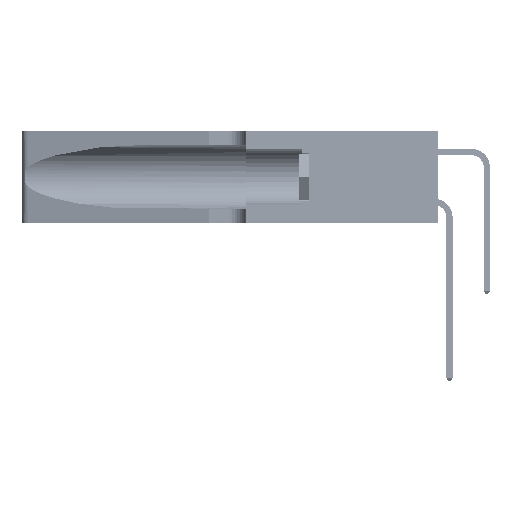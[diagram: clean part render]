
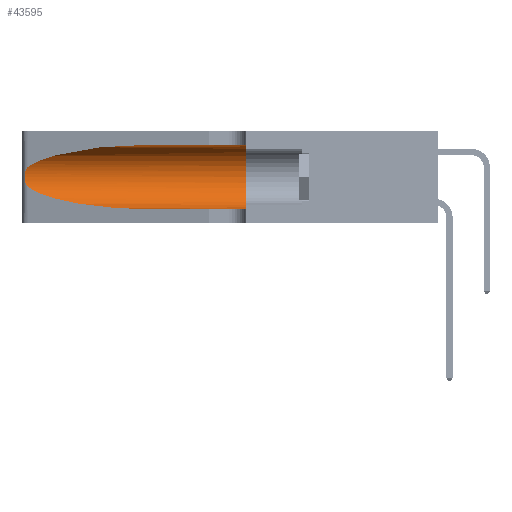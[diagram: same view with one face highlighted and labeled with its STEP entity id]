
A CAD part, left-side view. The second image highlights one B-rep face of the part: STEP entity #43595.
In plain terms, the highlighted cylindrical face has radius 3.308 mm (diameter 6.617 mm), a partial arc.
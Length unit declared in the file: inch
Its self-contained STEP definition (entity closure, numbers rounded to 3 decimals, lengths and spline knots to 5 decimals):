
#2756 = DIRECTION ( 'NONE',  ( 0., -1., 0. ) ) ;
#2828 = CARTESIAN_POINT ( 'NONE',  ( 0.26075, 1.23896, 0.19203 ) ) ;
#2876 = ORIENTED_EDGE ( 'NONE', *, *, #34880, .T. ) ;
#3377 = CARTESIAN_POINT ( 'NONE',  ( 0.2373, 1.15595, 0.28018 ) ) ;
#5323 = DIRECTION ( 'NONE',  ( 0., 1., 0. ) ) ;
#5921 =( BOUNDED_CURVE ( )  B_SPLINE_CURVE ( 3, ( #46669, #27201, #12002, #32480 ),
 .UNSPECIFIED., .F., .F. ) 
 B_SPLINE_CURVE_WITH_KNOTS ( ( 4, 4 ),
 ( 3.44316, 4.71239 ),
 .UNSPECIFIED. ) 
 CURVE ( )  GEOMETRIC_REPRESENTATION_ITEM ( )  RATIONAL_B_SPLINE_CURVE ( ( 1., 0.87, 0.87, 1. ) ) 
 REPRESENTATION_ITEM ( '' )  );
#6498 = DIRECTION ( 'NONE',  ( 0., 0., -1. ) ) ;
#6576 = CARTESIAN_POINT ( 'NONE',  ( 0.25787, 1.23484, 0.2124 ) ) ;
#6736 = CARTESIAN_POINT ( 'NONE',  ( 0.25856, 1.23593, 0.16098 ) ) ;
#7008 = CARTESIAN_POINT ( 'NONE',  ( 0.1305, 1.61858, 0.31525 ) ) ;
#7596 = EDGE_CURVE ( 'NONE', #20951, #20446, #5921, .T. ) ;
#8749 = ORIENTED_EDGE ( 'NONE', *, *, #7596, .T. ) ;
#9635 = ORIENTED_EDGE ( 'NONE', *, *, #31779, .F. ) ;
#11020 = FACE_OUTER_BOUND ( 'NONE', #47784, .T. ) ;
#11982 = AXIS2_PLACEMENT_3D ( 'NONE', #14523, #41685, #6498 ) ;
#12002 = CARTESIAN_POINT ( 'NONE',  ( 0.18966, 0.96281, 0.05475 ) ) ;
#12327 = CARTESIAN_POINT ( 'NONE',  ( 0.1305, 1.61858, 0.05475 ) ) ;
#14523 = CARTESIAN_POINT ( 'NONE',  ( 0.1305, 1.61858, 0.185 ) ) ;
#14598 = CARTESIAN_POINT ( 'NONE',  ( 0.25789, 1.23486, 0.15765 ) ) ;
#15685 = B_SPLINE_CURVE_WITH_KNOTS ( 'NONE', 3,
 ( #46182, #25860, #33729, #6576, #41766, #42127, #2828, #30127, #30470, #6736, #14598, #41951, #18509, #18688 ),
 .UNSPECIFIED., .F., .F.,
 ( 4, 2, 2, 2, 2, 2, 4 ),
 ( 0., 0.00027, 0.00053, 0.00107, 0.0016, 0.00187, 0.00214 ),
 .UNSPECIFIED. ) ;
#17091 = DIRECTION ( 'NONE',  ( 0., 0., 1. ) ) ;
#17261 = CARTESIAN_POINT ( 'NONE',  ( 0.1305, 0.35, 0.185 ) ) ;
#18509 = CARTESIAN_POINT ( 'NONE',  ( 0.25555, 1.22993, 0.14849 ) ) ;
#18688 = CARTESIAN_POINT ( 'NONE',  ( 0.25487, 1.22718, 0.14631 ) ) ;
#20446 = VERTEX_POINT ( 'NONE', #42704 ) ;
#20951 = VERTEX_POINT ( 'NONE', #38389 ) ;
#21345 = VECTOR ( 'NONE', #28200, 39.37008 ) ;
#22218 = VERTEX_POINT ( 'NONE', #33921 ) ;
#23157 = EDGE_CURVE ( 'NONE', #20446, #22218, #30506, .T. ) ;
#23649 = CARTESIAN_POINT ( 'NONE',  ( 0.1305, 0.72297, 0.31525 ) ) ;
#24875 = ORIENTED_EDGE ( 'NONE', *, *, #23157, .T. ) ;
#25860 = CARTESIAN_POINT ( 'NONE',  ( 0.25555, 1.22994, 0.2215 ) ) ;
#26998 = VECTOR ( 'NONE', #2756, 39.37008 ) ;
#27201 = CARTESIAN_POINT ( 'NONE',  ( 0.2373, 1.15595, 0.08982 ) ) ;
#27953 = EDGE_CURVE ( 'NONE', #42683, #32411, #41091, .T. ) ;
#28200 = DIRECTION ( 'NONE',  ( 0., -1., 0. ) ) ;
#29021 = AXIS2_PLACEMENT_3D ( 'NONE', #17261, #5323, #17091 ) ;
#30127 = CARTESIAN_POINT ( 'NONE',  ( 0.26075, 1.23896, 0.178 ) ) ;
#30178 = VERTEX_POINT ( 'NONE', #37545 ) ;
#30296 = EDGE_CURVE ( 'NONE', #42683, #30178, #35396, .T. ) ;
#30470 = CARTESIAN_POINT ( 'NONE',  ( 0.26017, 1.23833, 0.17102 ) ) ;
#30506 = LINE ( 'NONE', #12327, #21345 ) ;
#31779 = EDGE_CURVE ( 'NONE', #32411, #22218, #40630, .T. ) ;
#32411 = VERTEX_POINT ( 'NONE', #33432 ) ;
#32445 = ORIENTED_EDGE ( 'NONE', *, *, #30296, .T. ) ;
#32480 = CARTESIAN_POINT ( 'NONE',  ( 0.1305, 0.72297, 0.05475 ) ) ;
#33432 = CARTESIAN_POINT ( 'NONE',  ( 0.1305, 0.35, 0.31525 ) ) ;
#33729 = CARTESIAN_POINT ( 'NONE',  ( 0.25639, 1.23184, 0.21858 ) ) ;
#33921 = CARTESIAN_POINT ( 'NONE',  ( 0.1305, 0.35, 0.05475 ) ) ;
#34880 = EDGE_CURVE ( 'NONE', #30178, #20951, #15685, .T. ) ;
#35396 =( BOUNDED_CURVE ( )  B_SPLINE_CURVE ( 3, ( #50153, #38217, #3377, #42010 ),
 .UNSPECIFIED., .F., .T. ) 
 B_SPLINE_CURVE_WITH_KNOTS ( ( 4, 4 ),
 ( 1.5708, 2.84003 ),
 .UNSPECIFIED. ) 
 CURVE ( )  GEOMETRIC_REPRESENTATION_ITEM ( )  RATIONAL_B_SPLINE_CURVE ( ( 1., 0.87, 0.87, 1. ) ) 
 REPRESENTATION_ITEM ( '' )  );
#35874 = ORIENTED_EDGE ( 'NONE', *, *, #27953, .F. ) ;
#37545 = CARTESIAN_POINT ( 'NONE',  ( 0.25487, 1.22718, 0.22369 ) ) ;
#38217 = CARTESIAN_POINT ( 'NONE',  ( 0.18966, 0.96281, 0.31525 ) ) ;
#38389 = CARTESIAN_POINT ( 'NONE',  ( 0.25487, 1.22718, 0.14631 ) ) ;
#39771 = CYLINDRICAL_SURFACE ( 'NONE', #11982, 0.13025 ) ;
#40630 = CIRCLE ( 'NONE', #29021, 0.13025 ) ;
#41091 = LINE ( 'NONE', #7008, #26998 ) ;
#41685 = DIRECTION ( 'NONE',  ( 0., -1., 0. ) ) ;
#41766 = CARTESIAN_POINT ( 'NONE',  ( 0.25854, 1.2359, 0.20912 ) ) ;
#41951 = CARTESIAN_POINT ( 'NONE',  ( 0.25639, 1.23186, 0.15144 ) ) ;
#42010 = CARTESIAN_POINT ( 'NONE',  ( 0.25487, 1.22718, 0.22369 ) ) ;
#42127 = CARTESIAN_POINT ( 'NONE',  ( 0.26018, 1.23835, 0.19895 ) ) ;
#42683 = VERTEX_POINT ( 'NONE', #23649 ) ;
#42704 = CARTESIAN_POINT ( 'NONE',  ( 0.1305, 0.72297, 0.05475 ) ) ;
#43595 = ADVANCED_FACE ( 'NONE', ( #11020 ), #39771, .F. ) ;
#46182 = CARTESIAN_POINT ( 'NONE',  ( 0.25487, 1.22718, 0.22369 ) ) ;
#46669 = CARTESIAN_POINT ( 'NONE',  ( 0.25487, 1.22718, 0.14631 ) ) ;
#47784 = EDGE_LOOP ( 'NONE', ( #32445, #2876, #8749, #24875, #9635, #35874 ) ) ;
#50153 = CARTESIAN_POINT ( 'NONE',  ( 0.1305, 0.72297, 0.31525 ) ) ;
